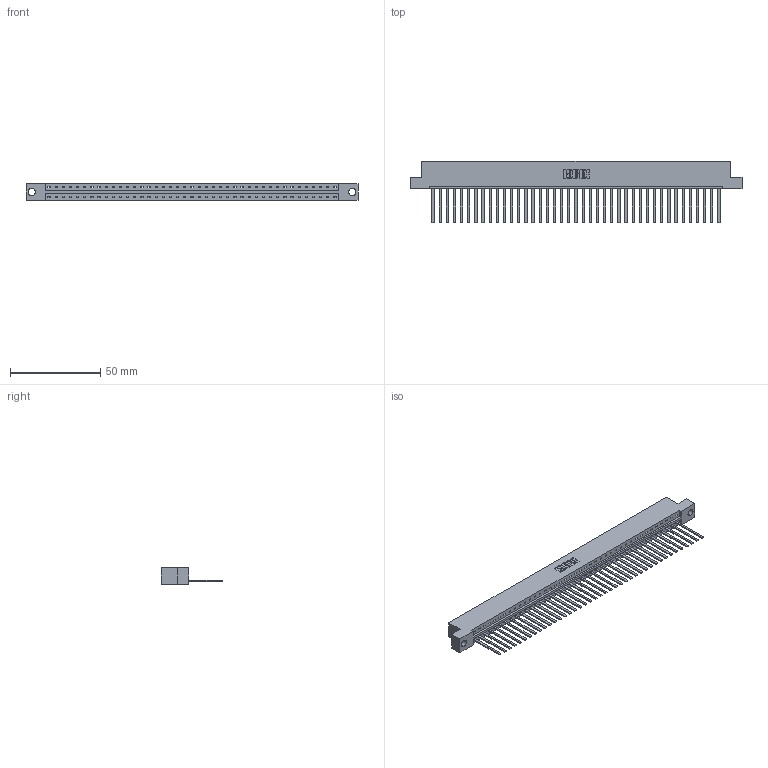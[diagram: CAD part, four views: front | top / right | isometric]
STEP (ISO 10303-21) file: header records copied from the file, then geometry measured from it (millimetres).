
FILE_DESCRIPTION (( 'STEP AP203' ), '1' );
FILE_NAME ('333-041-544-104.STEP', '2018-08-03T15:40:24', ( '' ), ( '' ), 'SwSTEP 2.0', 'SolidWorks 2016', '' );
FILE_SCHEMA (( 'CONFIG_CONTROL_DESIGN' ));
Length unit declared in the file: inch
Products named in the file (3): 333 Part_Flush - .156 Dia - TH; 345-292-001_345-293-144; 333-041-544-104
Assembly tree (42 placements, depth 2):
  333-041-544-104
    333 Part_Flush - .156 Dia - TH
    345-292-001_345-293-144  x41
Bounding box: 184 x 34.3 x 9.4 mm (x, y, z)
Volume: 18893.7 mm3; surface area: 21775.5 mm2
Topology: 42 solids, 42 shells, 2246 faces, 6789 edges, 4470 vertices
Faces by surface type: plane 1628, cylinder 618
Entity records: 25013 total; most frequent: CARTESIAN_POINT 4321, ORIENTED_EDGE 4298, DIRECTION 3643, EDGE_CURVE 2149, LINE 2025, VECTOR 2025, VERTEX_POINT 1430, AXIS2_PLACEMENT_3D 809
